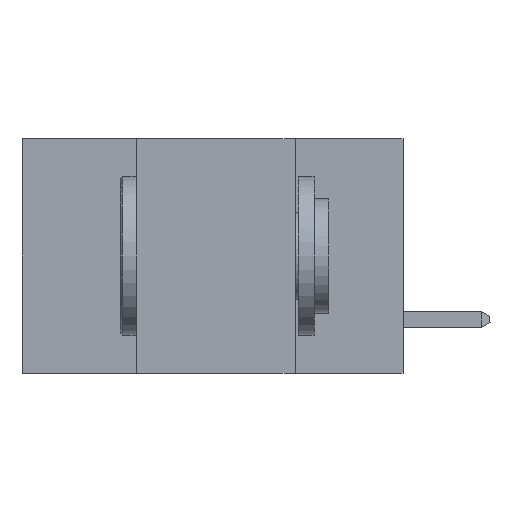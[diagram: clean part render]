
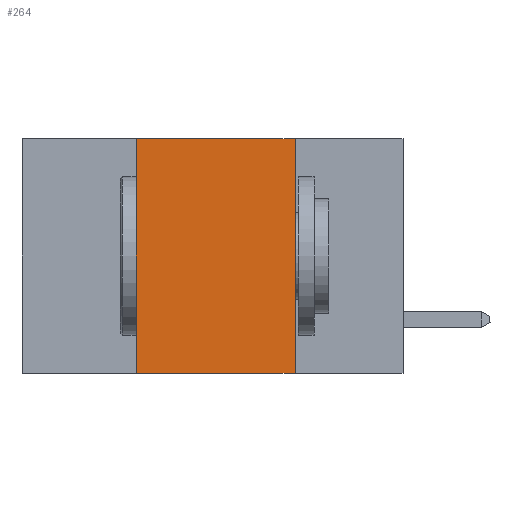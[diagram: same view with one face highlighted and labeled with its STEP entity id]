
A CAD part, left-side view. The second image highlights one B-rep face of the part: STEP entity #264.
In plain terms, the highlighted planar face has unit normal (-1, 0, 0).
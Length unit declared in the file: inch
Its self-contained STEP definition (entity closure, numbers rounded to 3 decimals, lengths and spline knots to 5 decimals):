
#264 = ADVANCED_FACE ( 'NONE', ( #4092 ), #14311, .F. ) ;
#503 = DIRECTION ( 'NONE',  ( 0., -1., 0. ) ) ;
#1833 = VERTEX_POINT ( 'NONE', #8707 ) ;
#2258 = EDGE_CURVE ( 'NONE', #1833, #7088, #6188, .T. ) ;
#2376 = AXIS2_PLACEMENT_3D ( 'NONE', #6145, #10295, #5966 ) ;
#2523 = CARTESIAN_POINT ( 'NONE',  ( 0., 0.6, 0. ) ) ;
#3153 = ORIENTED_EDGE ( 'NONE', *, *, #7326, .F. ) ;
#3239 = CARTESIAN_POINT ( 'NONE',  ( 0., 0.42, 0. ) ) ;
#3268 = CARTESIAN_POINT ( 'NONE',  ( 0., 0.42, 0. ) ) ;
#3873 = LINE ( 'NONE', #2523, #16189 ) ;
#4092 = FACE_OUTER_BOUND ( 'NONE', #6621, .T. ) ;
#4625 = CARTESIAN_POINT ( 'NONE',  ( 0., 0.17, 0. ) ) ;
#5204 = VERTEX_POINT ( 'NONE', #3239 ) ;
#5966 = DIRECTION ( 'NONE',  ( 0., 0., -1. ) ) ;
#6145 = CARTESIAN_POINT ( 'NONE',  ( 0., 0.6, 0. ) ) ;
#6188 = LINE ( 'NONE', #4625, #10076 ) ;
#6621 = EDGE_LOOP ( 'NONE', ( #16610, #3153, #15741, #16306 ) ) ;
#7088 = VERTEX_POINT ( 'NONE', #7760 ) ;
#7326 = EDGE_CURVE ( 'NONE', #5204, #1833, #3873, .T. ) ;
#7760 = CARTESIAN_POINT ( 'NONE',  ( 0., 0.17, -0.37 ) ) ;
#7913 = CARTESIAN_POINT ( 'NONE',  ( 0., 0.6, -0.37 ) ) ;
#8707 = CARTESIAN_POINT ( 'NONE',  ( 0., 0.17, 0. ) ) ;
#10076 = VECTOR ( 'NONE', #12689, 39.37008 ) ;
#10295 = DIRECTION ( 'NONE',  ( 1., 0., 0. ) ) ;
#10405 = VECTOR ( 'NONE', #14057, 39.37008 ) ;
#11323 = EDGE_CURVE ( 'NONE', #14415, #7088, #13991, .T. ) ;
#11534 = EDGE_CURVE ( 'NONE', #14415, #5204, #13760, .T. ) ;
#12054 = DIRECTION ( 'NONE',  ( 0., -1., 0. ) ) ;
#12689 = DIRECTION ( 'NONE',  ( 0., 0., -1. ) ) ;
#13760 = LINE ( 'NONE', #3268, #10405 ) ;
#13991 = LINE ( 'NONE', #7913, #16486 ) ;
#14057 = DIRECTION ( 'NONE',  ( 0., 0., 1. ) ) ;
#14311 = PLANE ( 'NONE',  #2376 ) ;
#14415 = VERTEX_POINT ( 'NONE', #16649 ) ;
#15741 = ORIENTED_EDGE ( 'NONE', *, *, #11534, .F. ) ;
#16189 = VECTOR ( 'NONE', #503, 39.37008 ) ;
#16306 = ORIENTED_EDGE ( 'NONE', *, *, #11323, .T. ) ;
#16486 = VECTOR ( 'NONE', #12054, 39.37008 ) ;
#16610 = ORIENTED_EDGE ( 'NONE', *, *, #2258, .F. ) ;
#16649 = CARTESIAN_POINT ( 'NONE',  ( 0., 0.42, -0.37 ) ) ;
